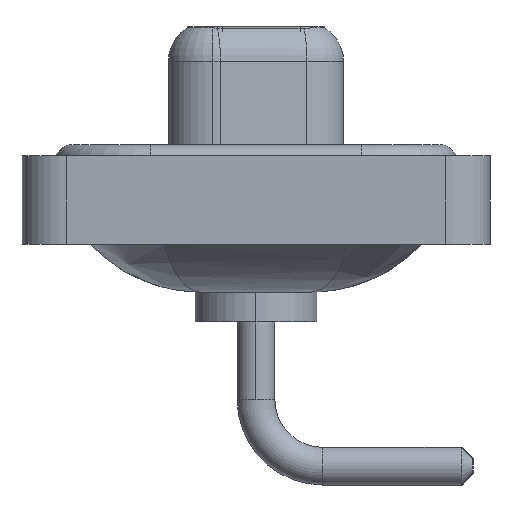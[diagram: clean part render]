
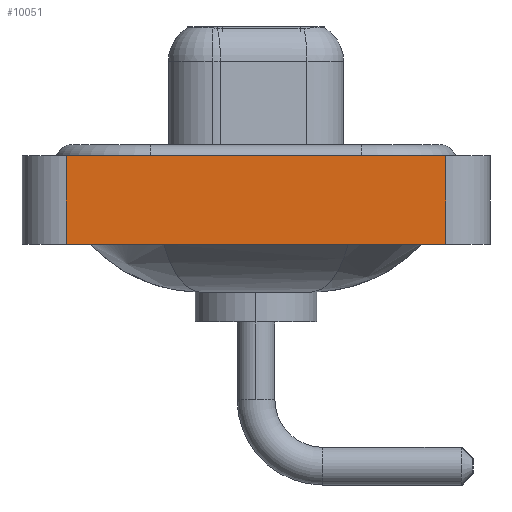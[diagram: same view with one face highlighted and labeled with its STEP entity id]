
A CAD part, left-side view. The second image highlights one B-rep face of the part: STEP entity #10051.
In plain terms, the highlighted planar face has unit normal (-1, 0, 0).
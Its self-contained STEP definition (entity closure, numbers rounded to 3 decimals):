
#91 = VECTOR ( 'NONE', #4081, 1000. ) ;
#640 = EDGE_CURVE ( 'NONE', #4412, #13970, #6229, .T. ) ;
#1197 = CARTESIAN_POINT ( 'NONE',  ( -7.3, -8.55, -3.6 ) ) ;
#2271 = FACE_OUTER_BOUND ( 'NONE', #11707, .T. ) ;
#2283 = VECTOR ( 'NONE', #14464, 1000. ) ;
#3050 = EDGE_CURVE ( 'NONE', #15751, #4412, #13731, .T. ) ;
#3524 = CARTESIAN_POINT ( 'NONE',  ( -7.3, -8.55, -3.6 ) ) ;
#3666 = LINE ( 'NONE', #13121, #13483 ) ;
#4081 = DIRECTION ( 'NONE',  ( 0., 0., 1. ) ) ;
#4247 = VERTEX_POINT ( 'NONE', #1197 ) ;
#4412 = VERTEX_POINT ( 'NONE', #8613 ) ;
#4884 = DIRECTION ( 'NONE',  ( 0., -1., 0. ) ) ;
#5222 = VECTOR ( 'NONE', #14116, 1000. ) ;
#5859 = CARTESIAN_POINT ( 'NONE',  ( -7.3, -8.55, -3.6 ) ) ;
#5975 = LINE ( 'NONE', #3524, #5222 ) ;
#6124 = PLANE ( 'NONE',  #14614 ) ;
#6229 = LINE ( 'NONE', #10241, #2283 ) ;
#7288 = ORIENTED_EDGE ( 'NONE', *, *, #3050, .F. ) ;
#8511 = CARTESIAN_POINT ( 'NONE',  ( -7.3, 8.55, -3.6 ) ) ;
#8613 = CARTESIAN_POINT ( 'NONE',  ( -7.3, 8.55, 0.4 ) ) ;
#8723 = DIRECTION ( 'NONE',  ( 0., 0., 1. ) ) ;
#9676 = CARTESIAN_POINT ( 'NONE',  ( -7.3, 8.55, -3.6 ) ) ;
#10051 = ADVANCED_FACE ( 'NONE', ( #2271 ), #6124, .T. ) ;
#10241 = CARTESIAN_POINT ( 'NONE',  ( -7.3, -8.55, 0.4 ) ) ;
#10640 = CARTESIAN_POINT ( 'NONE',  ( -7.3, -8.55, 0.4 ) ) ;
#10812 = ORIENTED_EDGE ( 'NONE', *, *, #14986, .T. ) ;
#11369 = DIRECTION ( 'NONE',  ( -1., 0., 0. ) ) ;
#11707 = EDGE_LOOP ( 'NONE', ( #15589, #11991, #7288, #10812 ) ) ;
#11991 = ORIENTED_EDGE ( 'NONE', *, *, #640, .F. ) ;
#12452 = EDGE_CURVE ( 'NONE', #4247, #13970, #5975, .T. ) ;
#13121 = CARTESIAN_POINT ( 'NONE',  ( -7.3, -8.55, -3.6 ) ) ;
#13483 = VECTOR ( 'NONE', #4884, 1000. ) ;
#13731 = LINE ( 'NONE', #9676, #91 ) ;
#13970 = VERTEX_POINT ( 'NONE', #10640 ) ;
#14116 = DIRECTION ( 'NONE',  ( 0., 0., 1. ) ) ;
#14464 = DIRECTION ( 'NONE',  ( 0., -1., 0. ) ) ;
#14614 = AXIS2_PLACEMENT_3D ( 'NONE', #5859, #11369, #8723 ) ;
#14986 = EDGE_CURVE ( 'NONE', #15751, #4247, #3666, .T. ) ;
#15589 = ORIENTED_EDGE ( 'NONE', *, *, #12452, .T. ) ;
#15751 = VERTEX_POINT ( 'NONE', #8511 ) ;
